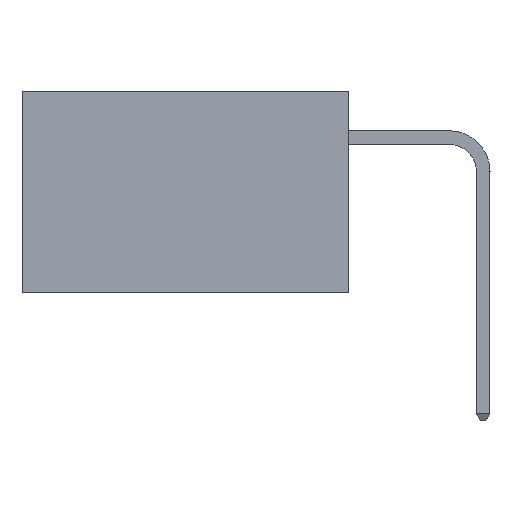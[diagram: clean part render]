
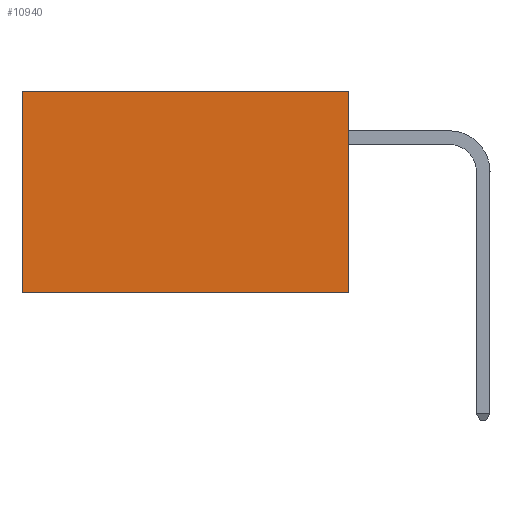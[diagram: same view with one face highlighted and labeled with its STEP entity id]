
A CAD part, left-side view. The second image highlights one B-rep face of the part: STEP entity #10940.
In plain terms, the highlighted planar face has unit normal (-1, 0, 0).
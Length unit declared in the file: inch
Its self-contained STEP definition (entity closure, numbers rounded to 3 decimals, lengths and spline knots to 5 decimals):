
#39 = CARTESIAN_POINT ( 'NONE',  ( 0.2875, 0., -0.37 ) ) ;
#290 = AXIS2_PLACEMENT_3D ( 'NONE', #9871, #16206, #8608 ) ;
#1407 = DIRECTION ( 'NONE',  ( 0., 0., -1. ) ) ;
#1572 = FACE_OUTER_BOUND ( 'NONE', #3221, .T. ) ;
#1879 = LINE ( 'NONE', #10235, #8304 ) ;
#2075 = CARTESIAN_POINT ( 'NONE',  ( 0.2875, 0.6, -0.37 ) ) ;
#2819 = EDGE_CURVE ( 'NONE', #7200, #4038, #6131, .T. ) ;
#3127 = DIRECTION ( 'NONE',  ( 0., 1., 0. ) ) ;
#3221 = EDGE_LOOP ( 'NONE', ( #13500, #12912, #14962, #5039 ) ) ;
#3764 = LINE ( 'NONE', #39, #16072 ) ;
#4038 = VERTEX_POINT ( 'NONE', #5562 ) ;
#4094 = EDGE_CURVE ( 'NONE', #7200, #4350, #1879, .T. ) ;
#4288 = CARTESIAN_POINT ( 'NONE',  ( 0.2875, 0., 0. ) ) ;
#4350 = VERTEX_POINT ( 'NONE', #11788 ) ;
#4357 = CARTESIAN_POINT ( 'NONE',  ( 0.2875, 0.6, 0. ) ) ;
#5039 = ORIENTED_EDGE ( 'NONE', *, *, #2819, .T. ) ;
#5562 = CARTESIAN_POINT ( 'NONE',  ( 0.2875, 0.6, 0. ) ) ;
#6131 = LINE ( 'NONE', #4288, #16312 ) ;
#6691 = EDGE_CURVE ( 'NONE', #4350, #15195, #3764, .T. ) ;
#7200 = VERTEX_POINT ( 'NONE', #14415 ) ;
#7307 = LINE ( 'NONE', #4357, #10768 ) ;
#8304 = VECTOR ( 'NONE', #1407, 39.37008 ) ;
#8608 = DIRECTION ( 'NONE',  ( 0., 0., -1. ) ) ;
#9871 = CARTESIAN_POINT ( 'NONE',  ( 0.2875, 0., 0. ) ) ;
#10235 = CARTESIAN_POINT ( 'NONE',  ( 0.2875, 0., 0. ) ) ;
#10768 = VECTOR ( 'NONE', #13251, 39.37008 ) ;
#10940 = ADVANCED_FACE ( 'NONE', ( #1572 ), #14957, .F. ) ;
#11788 = CARTESIAN_POINT ( 'NONE',  ( 0.2875, 0., -0.37 ) ) ;
#12912 = ORIENTED_EDGE ( 'NONE', *, *, #6691, .F. ) ;
#13251 = DIRECTION ( 'NONE',  ( 0., 0., -1. ) ) ;
#13500 = ORIENTED_EDGE ( 'NONE', *, *, #14460, .T. ) ;
#14415 = CARTESIAN_POINT ( 'NONE',  ( 0.2875, 0., 0. ) ) ;
#14460 = EDGE_CURVE ( 'NONE', #4038, #15195, #7307, .T. ) ;
#14957 = PLANE ( 'NONE',  #290 ) ;
#14962 = ORIENTED_EDGE ( 'NONE', *, *, #4094, .F. ) ;
#15195 = VERTEX_POINT ( 'NONE', #2075 ) ;
#15940 = DIRECTION ( 'NONE',  ( 0., 1., 0. ) ) ;
#16072 = VECTOR ( 'NONE', #3127, 39.37008 ) ;
#16206 = DIRECTION ( 'NONE',  ( 1., 0., 0. ) ) ;
#16312 = VECTOR ( 'NONE', #15940, 39.37008 ) ;
